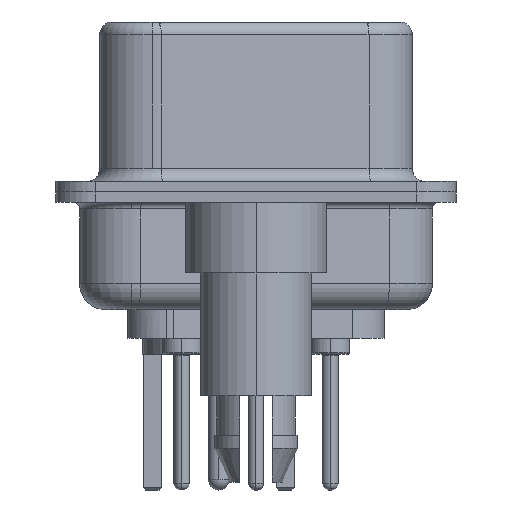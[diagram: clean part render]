
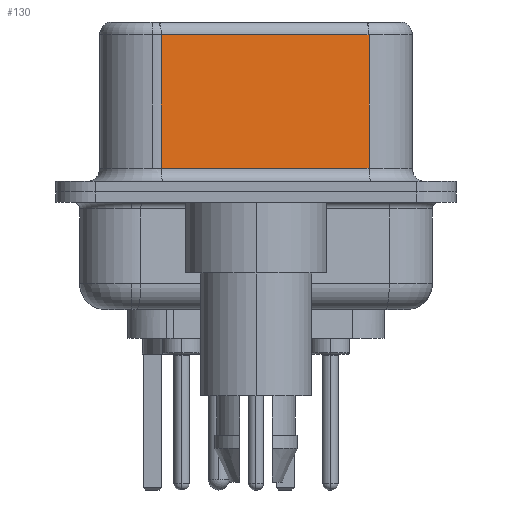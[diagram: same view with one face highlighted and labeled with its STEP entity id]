
A CAD part, left-side view. The second image highlights one B-rep face of the part: STEP entity #130.
In plain terms, the highlighted planar face has unit normal (-0.985, -0.174, 0).
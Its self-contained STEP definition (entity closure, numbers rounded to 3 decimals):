
#130 = ADVANCED_FACE ( 'NONE', ( #32549 ), #24613, .F. ) ;
#138 = VECTOR ( 'NONE', #35637, 1000. ) ;
#152 = EDGE_CURVE ( 'NONE', #12243, #34902, #16029, .T. ) ;
#1790 = AXIS2_PLACEMENT_3D ( 'NONE', #25463, #23830, #23591 ) ;
#2767 = EDGE_CURVE ( 'NONE', #22415, #12462, #27772, .T. ) ;
#3004 = CARTESIAN_POINT ( 'NONE',  ( 5.132, -4.322, 6.02 ) ) ;
#4191 = DIRECTION ( 'NONE',  ( 0., 0., -1. ) ) ;
#4297 = VECTOR ( 'NONE', #5762, 1000. ) ;
#5762 = DIRECTION ( 'NONE',  ( -0.174, 0.985, 0. ) ) ;
#6268 = ORIENTED_EDGE ( 'NONE', *, *, #9605, .T. ) ;
#7967 = CARTESIAN_POINT ( 'NONE',  ( 5.132, -4.322, 0.9 ) ) ;
#9605 = EDGE_CURVE ( 'NONE', #22415, #12243, #11709, .T. ) ;
#11709 = LINE ( 'NONE', #33411, #4297 ) ;
#12243 = VERTEX_POINT ( 'NONE', #16480 ) ;
#12462 = VERTEX_POINT ( 'NONE', #31425 ) ;
#16029 = LINE ( 'NONE', #22998, #23419 ) ;
#16480 = CARTESIAN_POINT ( 'NONE',  ( 3.73, 3.628, 6.02 ) ) ;
#19484 = VECTOR ( 'NONE', #4191, 1000. ) ;
#22415 = VERTEX_POINT ( 'NONE', #3004 ) ;
#22998 = CARTESIAN_POINT ( 'NONE',  ( 3.73, 3.628, 6.52 ) ) ;
#23233 = DIRECTION ( 'NONE',  ( 0., 0., -1. ) ) ;
#23419 = VECTOR ( 'NONE', #23233, 1000. ) ;
#23591 = DIRECTION ( 'NONE',  ( -0.174, 0.985, 0. ) ) ;
#23830 = DIRECTION ( 'NONE',  ( 0.985, 0.174, 0. ) ) ;
#24613 = PLANE ( 'NONE',  #1790 ) ;
#25463 = CARTESIAN_POINT ( 'NONE',  ( 5.132, -4.322, 6.52 ) ) ;
#27772 = LINE ( 'NONE', #28699, #19484 ) ;
#28699 = CARTESIAN_POINT ( 'NONE',  ( 5.132, -4.322, 6.52 ) ) ;
#28866 = ORIENTED_EDGE ( 'NONE', *, *, #2767, .F. ) ;
#29744 = LINE ( 'NONE', #7967, #138 ) ;
#30498 = CARTESIAN_POINT ( 'NONE',  ( 3.73, 3.628, 0.9 ) ) ;
#31425 = CARTESIAN_POINT ( 'NONE',  ( 5.132, -4.322, 0.9 ) ) ;
#32139 = EDGE_LOOP ( 'NONE', ( #28866, #6268, #35374, #34065 ) ) ;
#32549 = FACE_OUTER_BOUND ( 'NONE', #32139, .T. ) ;
#33411 = CARTESIAN_POINT ( 'NONE',  ( 5.132, -4.322, 6.02 ) ) ;
#34065 = ORIENTED_EDGE ( 'NONE', *, *, #35548, .T. ) ;
#34902 = VERTEX_POINT ( 'NONE', #30498 ) ;
#35374 = ORIENTED_EDGE ( 'NONE', *, *, #152, .T. ) ;
#35548 = EDGE_CURVE ( 'NONE', #34902, #12462, #29744, .T. ) ;
#35637 = DIRECTION ( 'NONE',  ( 0.174, -0.985, 0. ) ) ;
